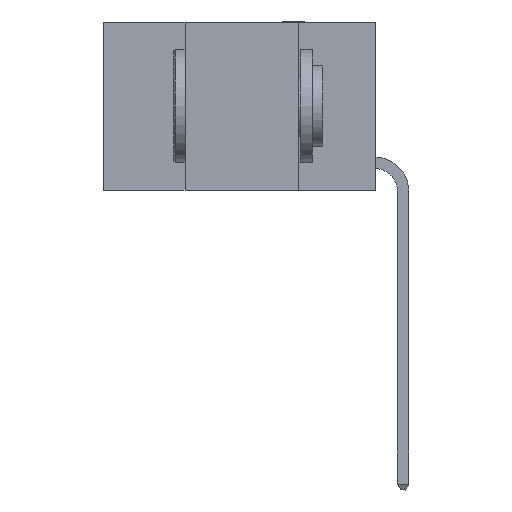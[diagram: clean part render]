
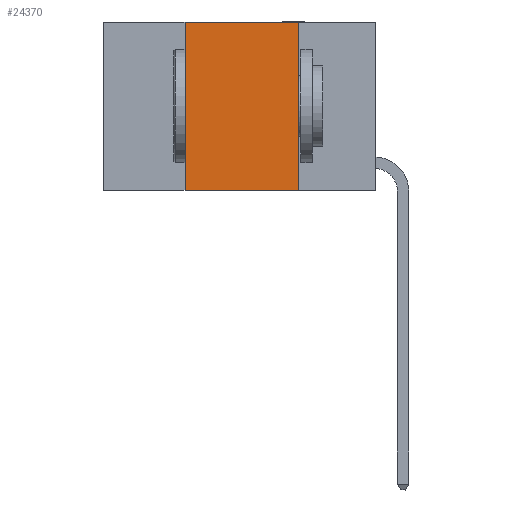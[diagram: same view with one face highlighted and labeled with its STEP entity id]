
A CAD part, left-side view. The second image highlights one B-rep face of the part: STEP entity #24370.
In plain terms, the highlighted planar face has unit normal (-1, 0, 0).
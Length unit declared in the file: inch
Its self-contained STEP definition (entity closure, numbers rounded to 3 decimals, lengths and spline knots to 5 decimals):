
#10 = CARTESIAN_POINT ( 'NONE',  ( 0., 0.6, -0.37 ) ) ;
#122 = EDGE_LOOP ( 'NONE', ( #1688, #15395, #25661, #9271 ) ) ;
#1016 = VECTOR ( 'NONE', #15848, 39.37008 ) ;
#1688 = ORIENTED_EDGE ( 'NONE', *, *, #23192, .F. ) ;
#1689 = FACE_OUTER_BOUND ( 'NONE', #122, .T. ) ;
#2888 = CARTESIAN_POINT ( 'NONE',  ( 0., 0.17, -0.37 ) ) ;
#3279 = DIRECTION ( 'NONE',  ( 0., -1., 0. ) ) ;
#4034 = DIRECTION ( 'NONE',  ( 0., -1., 0. ) ) ;
#5836 = AXIS2_PLACEMENT_3D ( 'NONE', #5848, #17869, #22003 ) ;
#5848 = CARTESIAN_POINT ( 'NONE',  ( 0., 0.6, 0. ) ) ;
#5885 = VECTOR ( 'NONE', #4034, 39.37008 ) ;
#7694 = CARTESIAN_POINT ( 'NONE',  ( 0., 0.42, 0. ) ) ;
#8107 = PLANE ( 'NONE',  #5836 ) ;
#8679 = VECTOR ( 'NONE', #3279, 39.37008 ) ;
#8895 = VERTEX_POINT ( 'NONE', #23962 ) ;
#9271 = ORIENTED_EDGE ( 'NONE', *, *, #23618, .T. ) ;
#9311 = CARTESIAN_POINT ( 'NONE',  ( 0., 0.6, 0. ) ) ;
#9891 = VERTEX_POINT ( 'NONE', #23528 ) ;
#11179 = LINE ( 'NONE', #9311, #8679 ) ;
#14199 = LINE ( 'NONE', #10, #5885 ) ;
#14694 = CARTESIAN_POINT ( 'NONE',  ( 0., 0.17, 0. ) ) ;
#15395 = ORIENTED_EDGE ( 'NONE', *, *, #19386, .F. ) ;
#15663 = VECTOR ( 'NONE', #20519, 39.37008 ) ;
#15848 = DIRECTION ( 'NONE',  ( 0., 0., 1. ) ) ;
#17869 = DIRECTION ( 'NONE',  ( 1., 0., 0. ) ) ;
#19386 = EDGE_CURVE ( 'NONE', #9891, #22835, #11179, .T. ) ;
#19435 = VERTEX_POINT ( 'NONE', #2888 ) ;
#19586 = EDGE_CURVE ( 'NONE', #8895, #9891, #25966, .T. ) ;
#20519 = DIRECTION ( 'NONE',  ( 0., 0., -1. ) ) ;
#22003 = DIRECTION ( 'NONE',  ( 0., 0., -1. ) ) ;
#22667 = LINE ( 'NONE', #24646, #15663 ) ;
#22835 = VERTEX_POINT ( 'NONE', #14694 ) ;
#23192 = EDGE_CURVE ( 'NONE', #22835, #19435, #22667, .T. ) ;
#23528 = CARTESIAN_POINT ( 'NONE',  ( 0., 0.42, 0. ) ) ;
#23618 = EDGE_CURVE ( 'NONE', #8895, #19435, #14199, .T. ) ;
#23962 = CARTESIAN_POINT ( 'NONE',  ( 0., 0.42, -0.37 ) ) ;
#24370 = ADVANCED_FACE ( 'NONE', ( #1689 ), #8107, .F. ) ;
#24646 = CARTESIAN_POINT ( 'NONE',  ( 0., 0.17, 0. ) ) ;
#25661 = ORIENTED_EDGE ( 'NONE', *, *, #19586, .F. ) ;
#25966 = LINE ( 'NONE', #7694, #1016 ) ;
